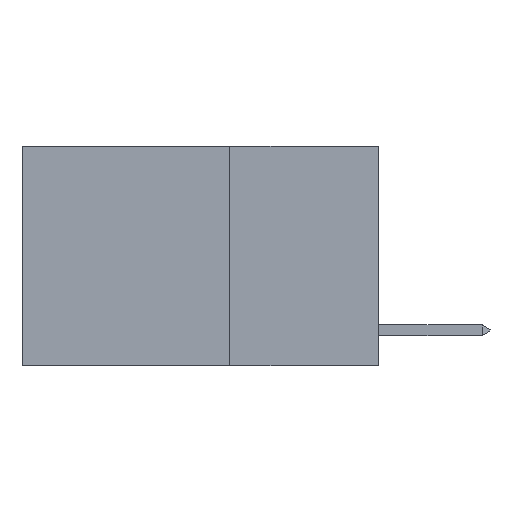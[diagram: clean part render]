
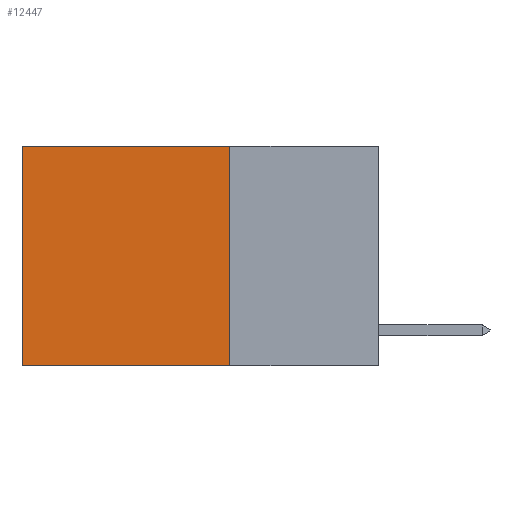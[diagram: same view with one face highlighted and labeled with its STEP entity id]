
A CAD part, left-side view. The second image highlights one B-rep face of the part: STEP entity #12447.
In plain terms, the highlighted planar face has unit normal (-1, 0, 0).
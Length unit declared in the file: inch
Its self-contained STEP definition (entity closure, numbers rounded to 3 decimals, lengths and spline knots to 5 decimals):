
#322 = CARTESIAN_POINT ( 'NONE',  ( 0.2625, 0.6, -0.37 ) ) ;
#852 = LINE ( 'NONE', #19353, #21860 ) ;
#1825 = EDGE_CURVE ( 'NONE', #3584, #6661, #11168, .T. ) ;
#2184 = VECTOR ( 'NONE', #4524, 39.37008 ) ;
#2650 = CARTESIAN_POINT ( 'NONE',  ( 0.2625, 0.25, 0. ) ) ;
#2959 = CARTESIAN_POINT ( 'NONE',  ( 0.2625, 0.25, 0. ) ) ;
#3584 = VERTEX_POINT ( 'NONE', #5927 ) ;
#4524 = DIRECTION ( 'NONE',  ( 0., 1., 0. ) ) ;
#5066 = CARTESIAN_POINT ( 'NONE',  ( 0.2625, 0.6, 0. ) ) ;
#5927 = CARTESIAN_POINT ( 'NONE',  ( 0.2625, 0.25, 0. ) ) ;
#6491 = AXIS2_PLACEMENT_3D ( 'NONE', #12860, #17593, #26012 ) ;
#6661 = VERTEX_POINT ( 'NONE', #23340 ) ;
#6987 = DIRECTION ( 'NONE',  ( 0., 0., -1. ) ) ;
#9047 = VECTOR ( 'NONE', #6987, 39.37008 ) ;
#9123 = FACE_OUTER_BOUND ( 'NONE', #25168, .T. ) ;
#9603 = ORIENTED_EDGE ( 'NONE', *, *, #21302, .T. ) ;
#11168 = LINE ( 'NONE', #2959, #14450 ) ;
#12072 = LINE ( 'NONE', #2650, #2184 ) ;
#12447 = ADVANCED_FACE ( 'NONE', ( #9123 ), #23310, .F. ) ;
#12860 = CARTESIAN_POINT ( 'NONE',  ( 0.2625, 0.25, 0. ) ) ;
#14450 = VECTOR ( 'NONE', #17629, 39.37008 ) ;
#16756 = CARTESIAN_POINT ( 'NONE',  ( 0.2625, 0.6, 0. ) ) ;
#16863 = ORIENTED_EDGE ( 'NONE', *, *, #27067, .T. ) ;
#17593 = DIRECTION ( 'NONE',  ( 1., 0., 0. ) ) ;
#17629 = DIRECTION ( 'NONE',  ( 0., 0., -1. ) ) ;
#18868 = VERTEX_POINT ( 'NONE', #16756 ) ;
#19353 = CARTESIAN_POINT ( 'NONE',  ( 0.2625, 0.25, -0.37 ) ) ;
#19365 = ORIENTED_EDGE ( 'NONE', *, *, #1825, .F. ) ;
#21302 = EDGE_CURVE ( 'NONE', #18868, #27094, #26365, .T. ) ;
#21860 = VECTOR ( 'NONE', #23668, 39.37008 ) ;
#23310 = PLANE ( 'NONE',  #6491 ) ;
#23340 = CARTESIAN_POINT ( 'NONE',  ( 0.2625, 0.25, -0.37 ) ) ;
#23668 = DIRECTION ( 'NONE',  ( 0., 1., 0. ) ) ;
#25168 = EDGE_LOOP ( 'NONE', ( #9603, #25266, #19365, #16863 ) ) ;
#25266 = ORIENTED_EDGE ( 'NONE', *, *, #27108, .F. ) ;
#26012 = DIRECTION ( 'NONE',  ( 0., 0., -1. ) ) ;
#26365 = LINE ( 'NONE', #5066, #9047 ) ;
#27067 = EDGE_CURVE ( 'NONE', #3584, #18868, #12072, .T. ) ;
#27094 = VERTEX_POINT ( 'NONE', #322 ) ;
#27108 = EDGE_CURVE ( 'NONE', #6661, #27094, #852, .T. ) ;
